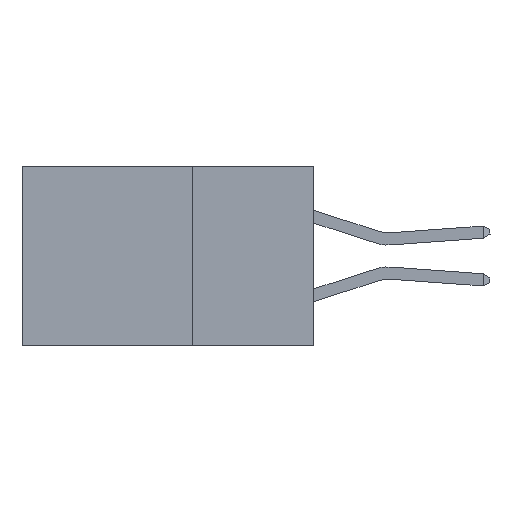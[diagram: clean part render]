
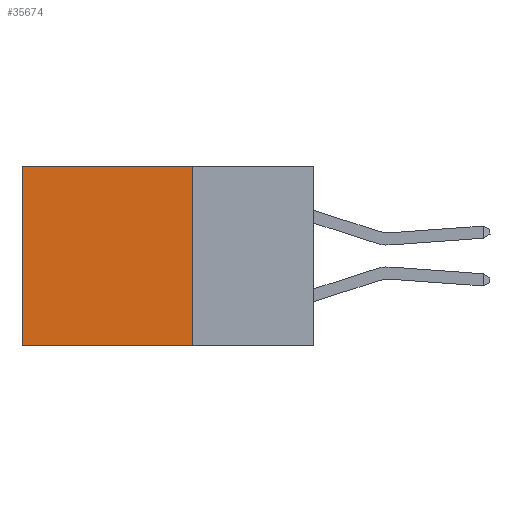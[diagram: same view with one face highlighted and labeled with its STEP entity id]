
A CAD part, left-side view. The second image highlights one B-rep face of the part: STEP entity #35674.
In plain terms, the highlighted planar face has unit normal (-1, 0, 0).
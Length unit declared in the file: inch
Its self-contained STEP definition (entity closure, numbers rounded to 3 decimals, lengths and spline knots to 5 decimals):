
#1560 = VERTEX_POINT ( 'NONE', #39335 ) ;
#3146 = LINE ( 'NONE', #10163, #41461 ) ;
#5456 = EDGE_CURVE ( 'NONE', #38343, #1560, #3146, .T. ) ;
#5752 = CARTESIAN_POINT ( 'NONE',  ( 0.2875, 0.25, 0. ) ) ;
#9516 = DIRECTION ( 'NONE',  ( 0., 1., 0. ) ) ;
#9548 = VECTOR ( 'NONE', #9516, 39.37008 ) ;
#9627 = DIRECTION ( 'NONE',  ( 1., 0., 0. ) ) ;
#10163 = CARTESIAN_POINT ( 'NONE',  ( 0.2875, 0.25, -0.37 ) ) ;
#11131 = EDGE_LOOP ( 'NONE', ( #32537, #42503, #42165, #13229 ) ) ;
#11901 = DIRECTION ( 'NONE',  ( 0., 0., -1. ) ) ;
#12162 = LINE ( 'NONE', #32279, #9548 ) ;
#13209 = VERTEX_POINT ( 'NONE', #42586 ) ;
#13229 = ORIENTED_EDGE ( 'NONE', *, *, #27913, .T. ) ;
#15072 = CARTESIAN_POINT ( 'NONE',  ( 0.2875, 0.6, 0. ) ) ;
#16185 = CARTESIAN_POINT ( 'NONE',  ( 0.2875, 0.25, 0. ) ) ;
#19770 = CARTESIAN_POINT ( 'NONE',  ( 0.2875, 0.25, -0.37 ) ) ;
#20557 = VERTEX_POINT ( 'NONE', #31030 ) ;
#20711 = VECTOR ( 'NONE', #28430, 39.37008 ) ;
#22990 = FACE_OUTER_BOUND ( 'NONE', #11131, .T. ) ;
#23077 = DIRECTION ( 'NONE',  ( 0., 1., 0. ) ) ;
#23277 = AXIS2_PLACEMENT_3D ( 'NONE', #16185, #9627, #36104 ) ;
#27913 = EDGE_CURVE ( 'NONE', #20557, #13209, #12162, .T. ) ;
#28430 = DIRECTION ( 'NONE',  ( 0., 0., -1. ) ) ;
#28544 = LINE ( 'NONE', #5752, #28759 ) ;
#28759 = VECTOR ( 'NONE', #11901, 39.37008 ) ;
#31030 = CARTESIAN_POINT ( 'NONE',  ( 0.2875, 0.25, 0. ) ) ;
#31066 = LINE ( 'NONE', #15072, #20711 ) ;
#32279 = CARTESIAN_POINT ( 'NONE',  ( 0.2875, 0.25, 0. ) ) ;
#32537 = ORIENTED_EDGE ( 'NONE', *, *, #39971, .T. ) ;
#34563 = EDGE_CURVE ( 'NONE', #20557, #38343, #28544, .T. ) ;
#35674 = ADVANCED_FACE ( 'NONE', ( #22990 ), #43102, .F. ) ;
#36104 = DIRECTION ( 'NONE',  ( 0., 0., -1. ) ) ;
#38343 = VERTEX_POINT ( 'NONE', #19770 ) ;
#39335 = CARTESIAN_POINT ( 'NONE',  ( 0.2875, 0.6, -0.37 ) ) ;
#39971 = EDGE_CURVE ( 'NONE', #13209, #1560, #31066, .T. ) ;
#41461 = VECTOR ( 'NONE', #23077, 39.37008 ) ;
#42165 = ORIENTED_EDGE ( 'NONE', *, *, #34563, .F. ) ;
#42503 = ORIENTED_EDGE ( 'NONE', *, *, #5456, .F. ) ;
#42586 = CARTESIAN_POINT ( 'NONE',  ( 0.2875, 0.6, 0. ) ) ;
#43102 = PLANE ( 'NONE',  #23277 ) ;
